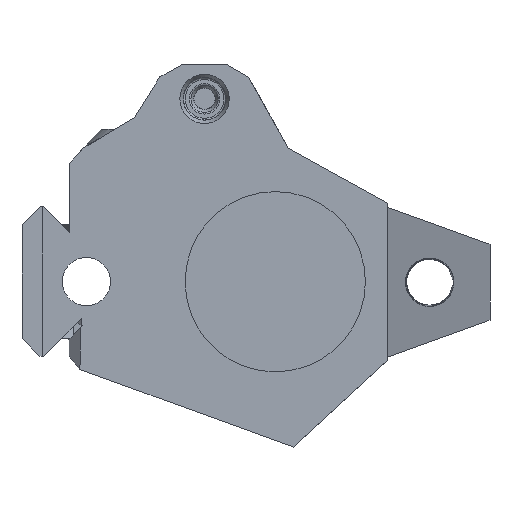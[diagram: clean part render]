
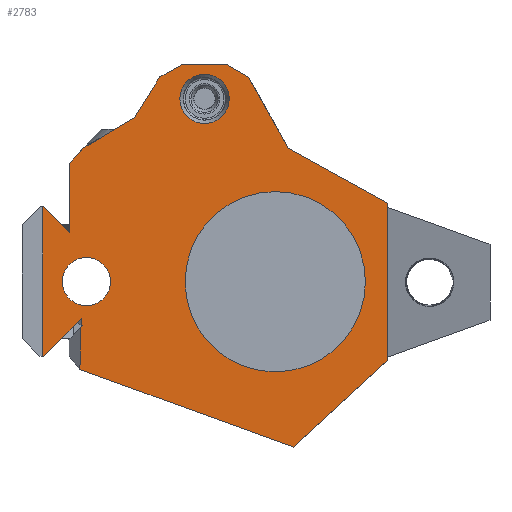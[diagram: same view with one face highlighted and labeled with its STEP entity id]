
A CAD part, left-side view. The second image highlights one B-rep face of the part: STEP entity #2783.
In plain terms, the highlighted planar face has unit normal (-1, 0, 0).
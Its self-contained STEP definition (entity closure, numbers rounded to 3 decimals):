
#54=PLANE('',#2989);
#167=FACE_BOUND('',#1036,.T.);
#168=FACE_BOUND('',#1037,.T.);
#169=FACE_BOUND('',#1038,.T.);
#224=LINE('',#4497,#535);
#227=LINE('',#4504,#538);
#228=LINE('',#4506,#539);
#229=LINE('',#4508,#540);
#230=LINE('',#4510,#541);
#231=LINE('',#4512,#542);
#232=LINE('',#4514,#543);
#233=LINE('',#4516,#544);
#234=LINE('',#4518,#545);
#235=LINE('',#4520,#546);
#236=LINE('',#4522,#547);
#237=LINE('',#4524,#548);
#238=LINE('',#4526,#549);
#239=LINE('',#4528,#550);
#240=LINE('',#4530,#551);
#241=LINE('',#4532,#552);
#242=LINE('',#4534,#553);
#243=LINE('',#4536,#554);
#244=LINE('',#4537,#555);
#245=LINE('',#4539,#556);
#246=LINE('',#4540,#557);
#535=VECTOR('',#3257,10.);
#538=VECTOR('',#3262,10.);
#539=VECTOR('',#3263,10.);
#540=VECTOR('',#3264,10.);
#541=VECTOR('',#3265,10.);
#542=VECTOR('',#3266,10.);
#543=VECTOR('',#3267,10.);
#544=VECTOR('',#3268,10.);
#545=VECTOR('',#3269,10.);
#546=VECTOR('',#3270,10.);
#547=VECTOR('',#3271,10.);
#548=VECTOR('',#3272,10.);
#549=VECTOR('',#3273,10.);
#550=VECTOR('',#3274,10.);
#551=VECTOR('',#3275,10.);
#552=VECTOR('',#3276,10.);
#553=VECTOR('',#3277,10.);
#554=VECTOR('',#3278,10.);
#555=VECTOR('',#3279,10.);
#556=VECTOR('',#3280,10.);
#557=VECTOR('',#3281,10.);
#873=FACE_OUTER_BOUND('',#1035,.T.);
#1035=EDGE_LOOP('',(#2028,#2029,#2030,#2031,#2032,#2033,#2034,#2035,#2036,
#2037,#2038,#2039,#2040,#2041,#2042,#2043,#2044,#2045,#2046,#2047,#2048));
#1036=EDGE_LOOP('',(#2049));
#1037=EDGE_LOOP('',(#2050));
#1038=EDGE_LOOP('',(#2051));
#1208=CIRCLE('',#2972,3.5);
#1219=CIRCLE('',#2990,12.773);
#1220=CIRCLE('',#2991,3.425);
#1259=VERTEX_POINT('',#4173);
#1271=VERTEX_POINT('',#4493);
#1273=VERTEX_POINT('',#4496);
#1275=VERTEX_POINT('',#4502);
#1276=VERTEX_POINT('',#4503);
#1277=VERTEX_POINT('',#4505);
#1278=VERTEX_POINT('',#4507);
#1279=VERTEX_POINT('',#4509);
#1280=VERTEX_POINT('',#4511);
#1281=VERTEX_POINT('',#4513);
#1282=VERTEX_POINT('',#4515);
#1283=VERTEX_POINT('',#4517);
#1284=VERTEX_POINT('',#4519);
#1285=VERTEX_POINT('',#4521);
#1286=VERTEX_POINT('',#4523);
#1287=VERTEX_POINT('',#4525);
#1288=VERTEX_POINT('',#4527);
#1289=VERTEX_POINT('',#4529);
#1290=VERTEX_POINT('',#4531);
#1291=VERTEX_POINT('',#4533);
#1292=VERTEX_POINT('',#4535);
#1293=VERTEX_POINT('',#4538);
#1294=VERTEX_POINT('',#4541);
#1295=VERTEX_POINT('',#4543);
#1539=EDGE_CURVE('',#1259,#1259,#1208,.T.);
#1560=EDGE_CURVE('',#1271,#1273,#224,.T.);
#1563=EDGE_CURVE('',#1275,#1276,#227,.T.);
#1564=EDGE_CURVE('',#1275,#1277,#228,.T.);
#1565=EDGE_CURVE('',#1277,#1278,#229,.T.);
#1566=EDGE_CURVE('',#1279,#1278,#230,.T.);
#1567=EDGE_CURVE('',#1280,#1279,#231,.T.);
#1568=EDGE_CURVE('',#1281,#1280,#232,.T.);
#1569=EDGE_CURVE('',#1282,#1281,#233,.T.);
#1570=EDGE_CURVE('',#1283,#1282,#234,.T.);
#1571=EDGE_CURVE('',#1284,#1283,#235,.T.);
#1572=EDGE_CURVE('',#1285,#1284,#236,.T.);
#1573=EDGE_CURVE('',#1286,#1285,#237,.F.);
#1574=EDGE_CURVE('',#1287,#1286,#238,.T.);
#1575=EDGE_CURVE('',#1288,#1287,#239,.T.);
#1576=EDGE_CURVE('',#1289,#1288,#240,.F.);
#1577=EDGE_CURVE('',#1290,#1289,#241,.T.);
#1578=EDGE_CURVE('',#1291,#1290,#242,.T.);
#1579=EDGE_CURVE('',#1292,#1291,#243,.T.);
#1580=EDGE_CURVE('',#1273,#1292,#244,.T.);
#1581=EDGE_CURVE('',#1293,#1271,#245,.T.);
#1582=EDGE_CURVE('',#1293,#1276,#246,.T.);
#1583=EDGE_CURVE('',#1294,#1294,#1219,.T.);
#1584=EDGE_CURVE('',#1295,#1295,#1220,.T.);
#2028=ORIENTED_EDGE('',*,*,#1563,.F.);
#2029=ORIENTED_EDGE('',*,*,#1564,.T.);
#2030=ORIENTED_EDGE('',*,*,#1565,.T.);
#2031=ORIENTED_EDGE('',*,*,#1566,.F.);
#2032=ORIENTED_EDGE('',*,*,#1567,.F.);
#2033=ORIENTED_EDGE('',*,*,#1568,.F.);
#2034=ORIENTED_EDGE('',*,*,#1569,.F.);
#2035=ORIENTED_EDGE('',*,*,#1570,.F.);
#2036=ORIENTED_EDGE('',*,*,#1571,.F.);
#2037=ORIENTED_EDGE('',*,*,#1572,.F.);
#2038=ORIENTED_EDGE('',*,*,#1573,.F.);
#2039=ORIENTED_EDGE('',*,*,#1574,.F.);
#2040=ORIENTED_EDGE('',*,*,#1575,.F.);
#2041=ORIENTED_EDGE('',*,*,#1576,.F.);
#2042=ORIENTED_EDGE('',*,*,#1577,.F.);
#2043=ORIENTED_EDGE('',*,*,#1578,.F.);
#2044=ORIENTED_EDGE('',*,*,#1579,.F.);
#2045=ORIENTED_EDGE('',*,*,#1580,.F.);
#2046=ORIENTED_EDGE('',*,*,#1560,.F.);
#2047=ORIENTED_EDGE('',*,*,#1581,.F.);
#2048=ORIENTED_EDGE('',*,*,#1582,.T.);
#2049=ORIENTED_EDGE('',*,*,#1583,.F.);
#2050=ORIENTED_EDGE('',*,*,#1584,.F.);
#2051=ORIENTED_EDGE('',*,*,#1539,.F.);
#2783=ADVANCED_FACE('',(#873,#167,#168,#169),#54,.T.);
#2972=AXIS2_PLACEMENT_3D('',#4174,#3219,#3220);
#2989=AXIS2_PLACEMENT_3D('',#4501,#3260,#3261);
#2990=AXIS2_PLACEMENT_3D('',#4542,#3282,#3283);
#2991=AXIS2_PLACEMENT_3D('',#4544,#3284,#3285);
#3219=DIRECTION('center_axis',(-1.,0.,0.));
#3220=DIRECTION('ref_axis',(0.,-1.,0.));
#3257=DIRECTION('',(0.,-0.489,-0.872));
#3260=DIRECTION('center_axis',(-1.,0.,0.));
#3261=DIRECTION('ref_axis',(0.,-1.,0.));
#3262=DIRECTION('',(0.,-0.875,0.484));
#3263=DIRECTION('',(0.,0.531,-0.847));
#3264=DIRECTION('',(0.,0.858,-0.513));
#3265=DIRECTION('',(0.,-0.669,0.743));
#3266=DIRECTION('',(0.,0.,1.));
#3267=DIRECTION('',(0.,-0.707,-0.707));
#3268=DIRECTION('',(0.,-0.924,0.383));
#3269=DIRECTION('',(0.,0.,1.));
#3270=DIRECTION('',(0.,1.,0.));
#3271=DIRECTION('',(0.,0.707,-0.707));
#3272=DIRECTION('',(0.,0.026,-1.));
#3273=DIRECTION('',(0.,0.864,0.504));
#3274=DIRECTION('',(0.,-0.707,0.707));
#3275=DIRECTION('',(0.,0.026,-1.));
#3276=DIRECTION('',(0.,0.94,0.342));
#3277=DIRECTION('',(0.,0.736,-0.677));
#3278=DIRECTION('',(0.,0.,-1.));
#3279=DIRECTION('',(0.,-0.875,-0.485));
#3280=DIRECTION('',(0.,-0.863,-0.505));
#3281=DIRECTION('',(0.,1.,0.));
#3282=DIRECTION('center_axis',(-1.,0.,0.));
#3283=DIRECTION('ref_axis',(0.,0.,
1.));
#3284=DIRECTION('center_axis',(-1.,0.,0.));
#3285=DIRECTION('ref_axis',(0.,-1.,0.));
#4173=CARTESIAN_POINT('',(587.112,197.565,-310.356));
#4174=CARTESIAN_POINT('Origin',(587.112,194.065,-310.356));
#4493=CARTESIAN_POINT('',(587.112,187.822,-307.3));
#4496=CARTESIAN_POINT('',(587.112,182.179,-317.362));
#4497=CARTESIAN_POINT('',(587.112,188.8,-305.556));
#4501=CARTESIAN_POINT('Origin',(587.112,192.573,-332.628));
#4502=CARTESIAN_POINT('',(587.112,200.392,-307.25));
#4503=CARTESIAN_POINT('',(587.112,197.329,-305.556));
#4504=CARTESIAN_POINT('',(587.112,202.007,-308.143));
#4505=CARTESIAN_POINT('',(587.112,204.,-313.));
#4506=CARTESIAN_POINT('',(587.112,204.469,-313.747));
#4507=CARTESIAN_POINT('',(587.112,211.294,-317.362));
#4508=CARTESIAN_POINT('',(587.112,204.115,-313.069));
#4509=CARTESIAN_POINT('',(587.112,213.201,-319.48));
#4510=CARTESIAN_POINT('',(587.112,210.38,-316.348));
#4511=CARTESIAN_POINT('',(587.112,213.201,-329.318));
#4512=CARTESIAN_POINT('',(587.112,213.201,-335.864));
#4513=CARTESIAN_POINT('',(587.112,216.905,-325.614));
#4514=CARTESIAN_POINT('',(587.112,195.411,-347.108));
#4515=CARTESIAN_POINT('',(587.112,217.011,-325.658));
#4516=CARTESIAN_POINT('',(587.112,206.397,-321.261));
#4517=CARTESIAN_POINT('',(587.112,217.011,-346.856));
#4518=CARTESIAN_POINT('',(587.112,217.011,-332.208));
#4519=CARTESIAN_POINT('',(587.112,216.872,-346.856));
#4520=CARTESIAN_POINT('',(587.112,201.822,-346.856));
#4521=CARTESIAN_POINT('',(587.112,211.545,-341.53));
#4522=CARTESIAN_POINT('',(587.112,206.251,-336.236));
#4523=CARTESIAN_POINT('',(587.112,211.567,-342.386));
#4524=CARTESIAN_POINT('',(587.112,211.626,-344.661));
#4525=CARTESIAN_POINT('',(587.112,211.335,-342.522));
#4526=CARTESIAN_POINT('',(587.112,202.769,-347.517));
#4527=CARTESIAN_POINT('',(587.112,211.577,-342.764));
#4528=CARTESIAN_POINT('',(587.112,196.303,-327.49));
#4529=CARTESIAN_POINT('',(587.112,211.729,-348.696));
#4530=CARTESIAN_POINT('',(587.112,211.626,-344.661));
#4531=CARTESIAN_POINT('',(587.112,181.497,-359.699));
#4532=CARTESIAN_POINT('',(587.112,189.884,-356.647));
#4533=CARTESIAN_POINT('',(587.112,168.134,-347.409));
#4534=CARTESIAN_POINT('',(587.112,177.799,-356.298));
#4535=CARTESIAN_POINT('',(587.112,168.134,-325.141));
#4536=CARTESIAN_POINT('',(587.112,168.134,-338.209));
#4537=CARTESIAN_POINT('',(587.112,178.878,-319.191));
#4538=CARTESIAN_POINT('',(587.112,190.8,-305.556));
#4539=CARTESIAN_POINT('',(587.112,184.812,-309.063));
#4540=CARTESIAN_POINT('',(587.112,191.951,-305.556));
#4541=CARTESIAN_POINT('',(587.112,184.042,-349.048));
#4542=CARTESIAN_POINT('Origin',(587.112,184.042,-336.275));
#4543=CARTESIAN_POINT('',(587.112,214.233,-336.252));
#4544=CARTESIAN_POINT('Origin',(587.112,210.808,-336.252));
